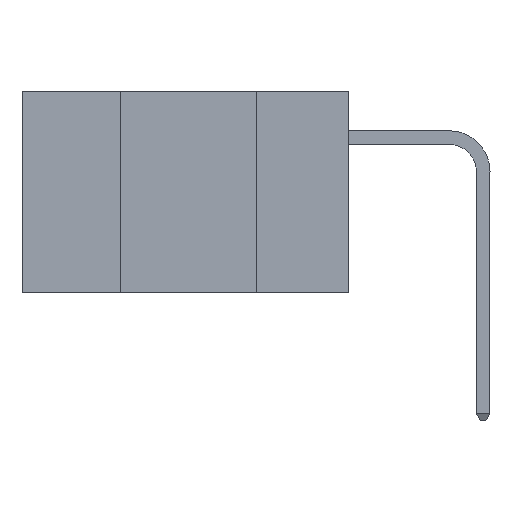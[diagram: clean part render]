
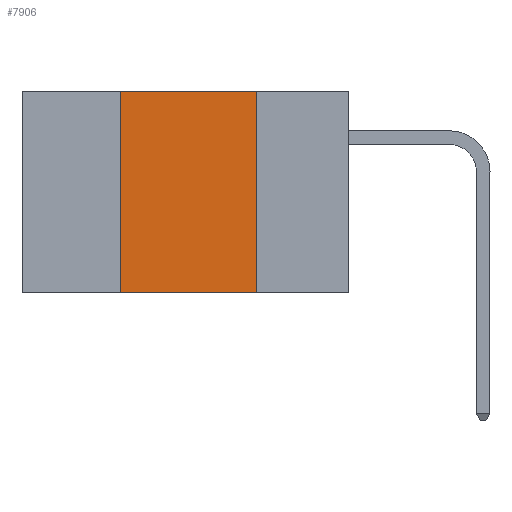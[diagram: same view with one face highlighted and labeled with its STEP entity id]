
A CAD part, left-side view. The second image highlights one B-rep face of the part: STEP entity #7906.
In plain terms, the highlighted planar face has unit normal (-1, 0, 0).
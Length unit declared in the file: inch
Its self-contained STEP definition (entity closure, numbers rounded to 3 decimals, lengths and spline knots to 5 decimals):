
#1139 = VECTOR ( 'NONE', #22412, 39.37008 ) ;
#1531 = VERTEX_POINT ( 'NONE', #2039 ) ;
#1597 = EDGE_CURVE ( 'NONE', #35823, #24407, #34524, .T. ) ;
#2016 = VECTOR ( 'NONE', #37426, 39.37008 ) ;
#2039 = CARTESIAN_POINT ( 'NONE',  ( 0., 0.17, -0.37 ) ) ;
#2224 = VERTEX_POINT ( 'NONE', #25440 ) ;
#7906 = ADVANCED_FACE ( 'NONE', ( #27025 ), #19876, .F. ) ;
#7961 = CARTESIAN_POINT ( 'NONE',  ( 0., 0.6, -0.37 ) ) ;
#8314 = EDGE_LOOP ( 'NONE', ( #34568, #15611, #9190, #26122 ) ) ;
#9190 = ORIENTED_EDGE ( 'NONE', *, *, #1597, .F. ) ;
#10456 = CARTESIAN_POINT ( 'NONE',  ( 0., 0.42, 0. ) ) ;
#11143 = DIRECTION ( 'NONE',  ( 1., 0., 0. ) ) ;
#11376 = VECTOR ( 'NONE', #19952, 39.37008 ) ;
#11454 = EDGE_CURVE ( 'NONE', #24407, #2224, #21015, .T. ) ;
#13016 = CARTESIAN_POINT ( 'NONE',  ( 0., 0.6, 0. ) ) ;
#13270 = VECTOR ( 'NONE', #16129, 39.37008 ) ;
#13362 = AXIS2_PLACEMENT_3D ( 'NONE', #28541, #11143, #31456 ) ;
#15333 = EDGE_CURVE ( 'NONE', #2224, #1531, #32942, .T. ) ;
#15611 = ORIENTED_EDGE ( 'NONE', *, *, #11454, .F. ) ;
#16129 = DIRECTION ( 'NONE',  ( 0., -1., 0. ) ) ;
#16736 = LINE ( 'NONE', #7961, #1139 ) ;
#19876 = PLANE ( 'NONE',  #13362 ) ;
#19952 = DIRECTION ( 'NONE',  ( 0., 0., 1. ) ) ;
#21015 = LINE ( 'NONE', #13016, #13270 ) ;
#21735 = CARTESIAN_POINT ( 'NONE',  ( 0., 0.42, -0.37 ) ) ;
#22412 = DIRECTION ( 'NONE',  ( 0., -1., 0. ) ) ;
#24407 = VERTEX_POINT ( 'NONE', #10456 ) ;
#25440 = CARTESIAN_POINT ( 'NONE',  ( 0., 0.17, 0. ) ) ;
#26122 = ORIENTED_EDGE ( 'NONE', *, *, #37349, .T. ) ;
#27025 = FACE_OUTER_BOUND ( 'NONE', #8314, .T. ) ;
#28541 = CARTESIAN_POINT ( 'NONE',  ( 0., 0.6, 0. ) ) ;
#31456 = DIRECTION ( 'NONE',  ( 0., 0., -1. ) ) ;
#32942 = LINE ( 'NONE', #34543, #2016 ) ;
#34524 = LINE ( 'NONE', #37205, #11376 ) ;
#34543 = CARTESIAN_POINT ( 'NONE',  ( 0., 0.17, 0. ) ) ;
#34568 = ORIENTED_EDGE ( 'NONE', *, *, #15333, .F. ) ;
#35823 = VERTEX_POINT ( 'NONE', #21735 ) ;
#37205 = CARTESIAN_POINT ( 'NONE',  ( 0., 0.42, 0. ) ) ;
#37349 = EDGE_CURVE ( 'NONE', #35823, #1531, #16736, .T. ) ;
#37426 = DIRECTION ( 'NONE',  ( 0., 0., -1. ) ) ;
